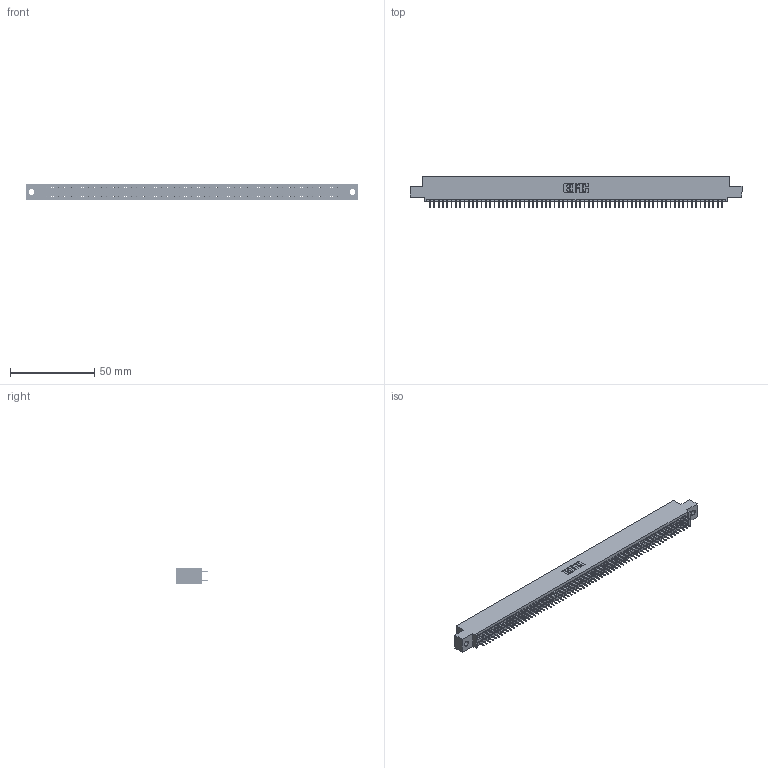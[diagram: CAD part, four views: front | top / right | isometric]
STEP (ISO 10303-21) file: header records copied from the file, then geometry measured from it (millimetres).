
FILE_DESCRIPTION (( 'STEP AP203' ), '1' );
FILE_NAME ('395-138-525-502.STEP', '2020-09-26T04:55:11', ( '' ), ( '' ), 'SwSTEP 2.0', 'SolidWorks 2020', '' );
FILE_SCHEMA (( 'CONFIG_CONTROL_DESIGN' ));
Length unit declared in the file: inch
Products named in the file (3): 345 Part_0.110 Offset - 0.128 Dia; 345-292-001_345-293-125; 395-138-525-502
Assembly tree (139 placements, depth 2):
  395-138-525-502
    345 Part_0.110 Offset - 0.128 Dia
    345-292-001_345-293-125  x138
Bounding box: 196.47 x 18.72 x 9.4 mm (x, y, z)
Volume: 18998.6 mm3; surface area: 27741.7 mm2
Topology: 139 solids, 139 shells, 7582 faces, 21467 edges, 13758 vertices
Faces by surface type: plane 5466, cylinder 2116
Entity records: 50713 total; most frequent: CARTESIAN_POINT 8476, ORIENTED_EDGE 8410, DIRECTION 7441, EDGE_CURVE 4205, LINE 3801, VECTOR 3801, VERTEX_POINT 2798, AXIS2_PLACEMENT_3D 1820
